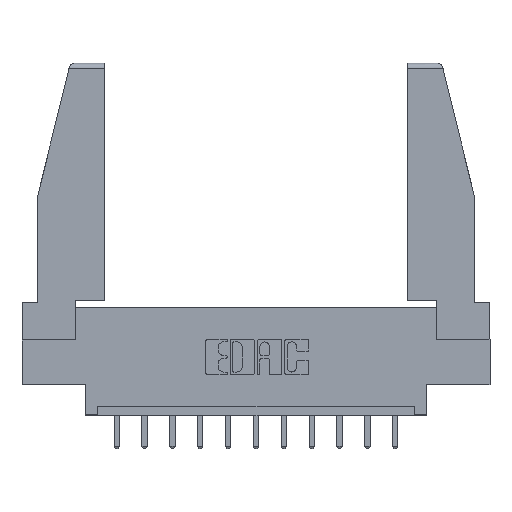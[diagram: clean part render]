
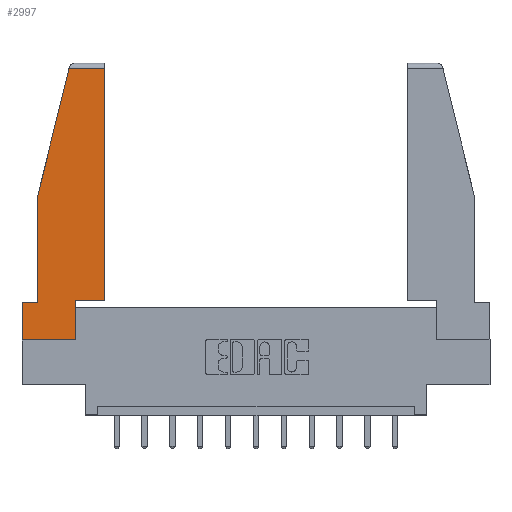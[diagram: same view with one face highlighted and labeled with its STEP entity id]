
A CAD part, top view. The second image highlights one B-rep face of the part: STEP entity #2997.
In plain terms, the highlighted planar face has unit normal (0, 0, 1).
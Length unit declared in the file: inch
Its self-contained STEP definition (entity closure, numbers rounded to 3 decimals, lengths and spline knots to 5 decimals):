
#161 = EDGE_CURVE ( 'NONE', #14604, #3810, #10336, .T. ) ;
#172 = CARTESIAN_POINT ( 'NONE',  ( 0.086, 0.8, 0. ) ) ;
#333 = VERTEX_POINT ( 'NONE', #6703 ) ;
#456 = ORIENTED_EDGE ( 'NONE', *, *, #861, .T. ) ;
#861 = EDGE_CURVE ( 'NONE', #333, #11678, #4563, .T. ) ;
#1177 = VECTOR ( 'NONE', #8190, 39.37008 ) ;
#1281 = VECTOR ( 'NONE', #7200, 39.37008 ) ;
#1336 = LINE ( 'NONE', #13021, #13204 ) ;
#1357 = VECTOR ( 'NONE', #8556, 39.37008 ) ;
#1708 = CARTESIAN_POINT ( 'NONE',  ( 0.297, 0., 0. ) ) ;
#1712 = LINE ( 'NONE', #1708, #12006 ) ;
#2071 = CARTESIAN_POINT ( 'NONE',  ( 0.2636, 1.52, 0. ) ) ;
#2134 = VECTOR ( 'NONE', #5601, 39.37008 ) ;
#2149 = CARTESIAN_POINT ( 'NONE',  ( 0., 0., 0. ) ) ;
#2159 = DIRECTION ( 'NONE',  ( -0.239, -0.971, 0. ) ) ;
#2225 = CARTESIAN_POINT ( 'NONE',  ( 0.086, 0.21, 0. ) ) ;
#2363 = LINE ( 'NONE', #13379, #3070 ) ;
#2449 = EDGE_CURVE ( 'NONE', #11678, #12778, #10348, .T. ) ;
#2587 = ORIENTED_EDGE ( 'NONE', *, *, #2700, .T. ) ;
#2700 = EDGE_CURVE ( 'NONE', #13744, #4212, #1336, .T. ) ;
#2997 = ADVANCED_FACE ( 'NONE', ( #4198 ), #12542, .T. ) ;
#3045 = EDGE_CURVE ( 'NONE', #12778, #14604, #9465, .T. ) ;
#3070 = VECTOR ( 'NONE', #8842, 39.37008 ) ;
#3810 = VERTEX_POINT ( 'NONE', #172 ) ;
#4198 = FACE_OUTER_BOUND ( 'NONE', #10006, .T. ) ;
#4212 = VERTEX_POINT ( 'NONE', #8453 ) ;
#4563 = LINE ( 'NONE', #9690, #12664 ) ;
#4912 = CARTESIAN_POINT ( 'NONE',  ( 0., 0., 0. ) ) ;
#5335 = CARTESIAN_POINT ( 'NONE',  ( 0.086, 0.8, 0. ) ) ;
#5370 = ORIENTED_EDGE ( 'NONE', *, *, #161, .T. ) ;
#5601 = DIRECTION ( 'NONE',  ( 0., -1., 0. ) ) ;
#5604 = CARTESIAN_POINT ( 'NONE',  ( 0.271, 1.55, 0. ) ) ;
#5672 = AXIS2_PLACEMENT_3D ( 'NONE', #2149, #7891, #11387 ) ;
#5891 = CARTESIAN_POINT ( 'NONE',  ( 0., 1.52, 0. ) ) ;
#6509 = CARTESIAN_POINT ( 'NONE',  ( 0.461, 1.52, 0. ) ) ;
#6703 = CARTESIAN_POINT ( 'NONE',  ( 0.297, 0.223, 0. ) ) ;
#7064 = LINE ( 'NONE', #4912, #1281 ) ;
#7067 = ORIENTED_EDGE ( 'NONE', *, *, #14908, .T. ) ;
#7200 = DIRECTION ( 'NONE',  ( 1., 0., 0. ) ) ;
#7364 = ORIENTED_EDGE ( 'NONE', *, *, #10052, .T. ) ;
#7701 = CARTESIAN_POINT ( 'NONE',  ( 0.297, 0., 0. ) ) ;
#7891 = DIRECTION ( 'NONE',  ( 0., 0., 1. ) ) ;
#8043 = VECTOR ( 'NONE', #2159, 39.37008 ) ;
#8190 = DIRECTION ( 'NONE',  ( -1., 0., 0. ) ) ;
#8280 = ORIENTED_EDGE ( 'NONE', *, *, #8479, .T. ) ;
#8453 = CARTESIAN_POINT ( 'NONE',  ( 0., 0.21, 0. ) ) ;
#8479 = EDGE_CURVE ( 'NONE', #4212, #12242, #2363, .T. ) ;
#8556 = DIRECTION ( 'NONE',  ( 0., 1., 0. ) ) ;
#8575 = DIRECTION ( 'NONE',  ( 1., 0., 0. ) ) ;
#8637 = DIRECTION ( 'NONE',  ( -1., 0., 0. ) ) ;
#8842 = DIRECTION ( 'NONE',  ( 0., -1., 0. ) ) ;
#9404 = VERTEX_POINT ( 'NONE', #7701 ) ;
#9465 = LINE ( 'NONE', #5891, #1177 ) ;
#9690 = CARTESIAN_POINT ( 'NONE',  ( 0.297, 0.223, 0. ) ) ;
#9775 = DIRECTION ( 'NONE',  ( 0., 1., 0. ) ) ;
#9893 = CARTESIAN_POINT ( 'NONE',  ( 0., 0., 0. ) ) ;
#10006 = EDGE_LOOP ( 'NONE', ( #14437, #12559, #5370, #7364, #2587, #8280, #7067, #11385, #456 ) ) ;
#10052 = EDGE_CURVE ( 'NONE', #3810, #13744, #14020, .T. ) ;
#10336 = LINE ( 'NONE', #5604, #8043 ) ;
#10348 = LINE ( 'NONE', #10931, #1357 ) ;
#10931 = CARTESIAN_POINT ( 'NONE',  ( 0.461, 0.223, 0. ) ) ;
#11385 = ORIENTED_EDGE ( 'NONE', *, *, #11543, .T. ) ;
#11387 = DIRECTION ( 'NONE',  ( 1., 0., 0. ) ) ;
#11543 = EDGE_CURVE ( 'NONE', #9404, #333, #1712, .T. ) ;
#11678 = VERTEX_POINT ( 'NONE', #12727 ) ;
#12006 = VECTOR ( 'NONE', #9775, 39.37008 ) ;
#12242 = VERTEX_POINT ( 'NONE', #9893 ) ;
#12542 = PLANE ( 'NONE',  #5672 ) ;
#12559 = ORIENTED_EDGE ( 'NONE', *, *, #3045, .T. ) ;
#12664 = VECTOR ( 'NONE', #8575, 39.37008 ) ;
#12727 = CARTESIAN_POINT ( 'NONE',  ( 0.461, 0.223, 0. ) ) ;
#12778 = VERTEX_POINT ( 'NONE', #6509 ) ;
#13021 = CARTESIAN_POINT ( 'NONE',  ( 0., 0.21, 0. ) ) ;
#13204 = VECTOR ( 'NONE', #8637, 39.37008 ) ;
#13379 = CARTESIAN_POINT ( 'NONE',  ( 0., 0.21, 0. ) ) ;
#13744 = VERTEX_POINT ( 'NONE', #2225 ) ;
#14020 = LINE ( 'NONE', #5335, #2134 ) ;
#14437 = ORIENTED_EDGE ( 'NONE', *, *, #2449, .T. ) ;
#14604 = VERTEX_POINT ( 'NONE', #2071 ) ;
#14908 = EDGE_CURVE ( 'NONE', #12242, #9404, #7064, .T. ) ;
